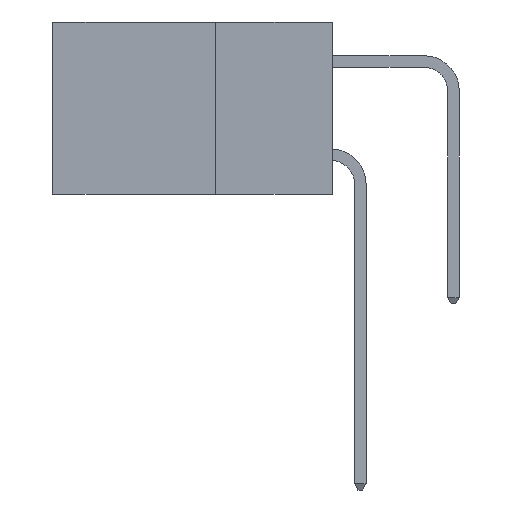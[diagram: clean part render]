
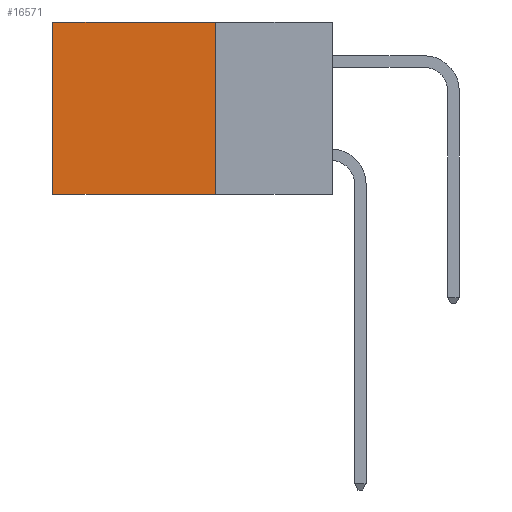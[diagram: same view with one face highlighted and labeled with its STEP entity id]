
A CAD part, left-side view. The second image highlights one B-rep face of the part: STEP entity #16571.
In plain terms, the highlighted planar face has unit normal (-1, 0, 0).
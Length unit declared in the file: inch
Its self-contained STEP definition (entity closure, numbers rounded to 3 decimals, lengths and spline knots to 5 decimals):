
#458 = DIRECTION ( 'NONE',  ( 0., 0., -1. ) ) ;
#627 = ORIENTED_EDGE ( 'NONE', *, *, #18041, .F. ) ;
#1659 = LINE ( 'NONE', #16573, #16423 ) ;
#2031 = VERTEX_POINT ( 'NONE', #5501 ) ;
#2437 = CARTESIAN_POINT ( 'NONE',  ( 0.2615, 0.6, -0.37 ) ) ;
#3979 = AXIS2_PLACEMENT_3D ( 'NONE', #8061, #9535, #458 ) ;
#4074 = EDGE_LOOP ( 'NONE', ( #4075, #627, #15041, #10995 ) ) ;
#4075 = ORIENTED_EDGE ( 'NONE', *, *, #9368, .T. ) ;
#4977 = VERTEX_POINT ( 'NONE', #14941 ) ;
#5501 = CARTESIAN_POINT ( 'NONE',  ( 0.2615, 0.6, 0. ) ) ;
#5597 = VERTEX_POINT ( 'NONE', #7463 ) ;
#5932 = DIRECTION ( 'NONE',  ( 0., 1., 0. ) ) ;
#6777 = DIRECTION ( 'NONE',  ( 0., 0., -1. ) ) ;
#7463 = CARTESIAN_POINT ( 'NONE',  ( 0.2615, 0.25, 0. ) ) ;
#8061 = CARTESIAN_POINT ( 'NONE',  ( 0.2615, 0.25, -0.37 ) ) ;
#8335 = VECTOR ( 'NONE', #5932, 39.37008 ) ;
#9368 = EDGE_CURVE ( 'NONE', #2031, #18050, #1659, .T. ) ;
#9417 = DIRECTION ( 'NONE',  ( 0., 0., -1. ) ) ;
#9535 = DIRECTION ( 'NONE',  ( 1., 0., 0. ) ) ;
#10995 = ORIENTED_EDGE ( 'NONE', *, *, #15034, .T. ) ;
#11346 = CARTESIAN_POINT ( 'NONE',  ( 0.2615, 0.25, -0.37 ) ) ;
#12115 = LINE ( 'NONE', #16091, #8335 ) ;
#12335 = VECTOR ( 'NONE', #6777, 39.37008 ) ;
#12809 = DIRECTION ( 'NONE',  ( 0., 1., 0. ) ) ;
#14553 = VECTOR ( 'NONE', #12809, 39.37008 ) ;
#14941 = CARTESIAN_POINT ( 'NONE',  ( 0.2615, 0.25, -0.37 ) ) ;
#15034 = EDGE_CURVE ( 'NONE', #5597, #2031, #12115, .T. ) ;
#15041 = ORIENTED_EDGE ( 'NONE', *, *, #15307, .F. ) ;
#15307 = EDGE_CURVE ( 'NONE', #5597, #4977, #16200, .T. ) ;
#15443 = CARTESIAN_POINT ( 'NONE',  ( 0.2615, 0.25, -0.37 ) ) ;
#16091 = CARTESIAN_POINT ( 'NONE',  ( 0.2615, 0.25, 0. ) ) ;
#16200 = LINE ( 'NONE', #15443, #12335 ) ;
#16423 = VECTOR ( 'NONE', #9417, 39.37008 ) ;
#16571 = ADVANCED_FACE ( 'NONE', ( #16845 ), #16690, .F. ) ;
#16573 = CARTESIAN_POINT ( 'NONE',  ( 0.2615, 0.6, -0.37 ) ) ;
#16690 = PLANE ( 'NONE',  #3979 ) ;
#16845 = FACE_OUTER_BOUND ( 'NONE', #4074, .T. ) ;
#18041 = EDGE_CURVE ( 'NONE', #4977, #18050, #18785, .T. ) ;
#18050 = VERTEX_POINT ( 'NONE', #2437 ) ;
#18785 = LINE ( 'NONE', #11346, #14553 ) ;
